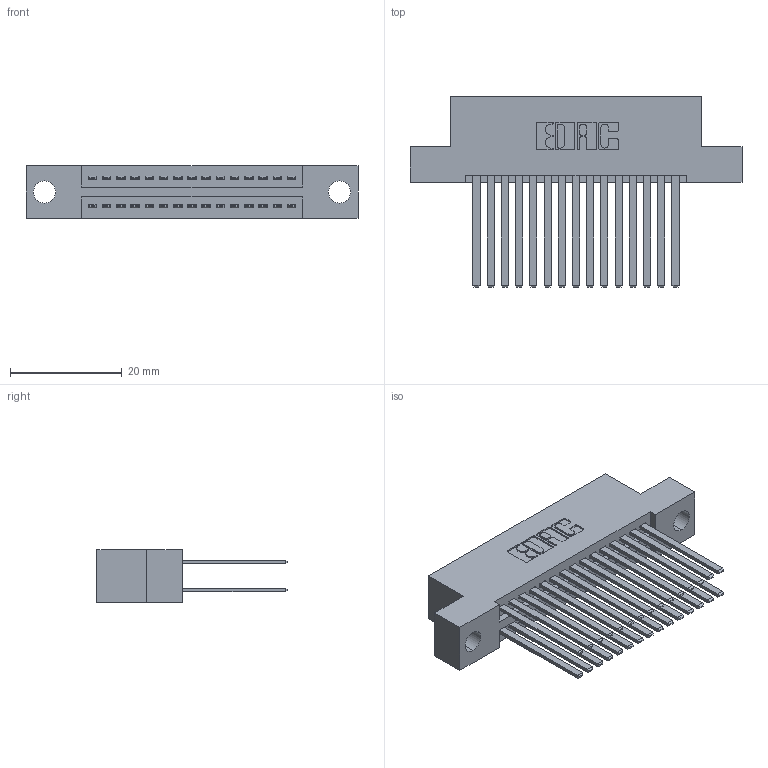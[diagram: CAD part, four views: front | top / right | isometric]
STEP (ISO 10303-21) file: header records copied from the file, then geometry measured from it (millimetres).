
FILE_DESCRIPTION (( 'STEP AP203' ), '1' );
FILE_NAME ('345-030-544-204.STEP', '2021-05-19T23:26:28', ( '' ), ( '' ), 'SwSTEP 2.0', 'SolidWorks 2020', '' );
FILE_SCHEMA (( 'CONFIG_CONTROL_DESIGN' ));
Length unit declared in the file: inch
Products named in the file (3): 345-292-001_345-293-144; 345 Part_Flush Mounting Lugs - 0.156 Dia-TI; 345-030-544-204
Assembly tree (31 placements, depth 2):
  345-030-544-204
    345 Part_Flush Mounting Lugs - 0.156 Dia-TI
    345-292-001_345-293-144  x30
Bounding box: 59.31 x 33.96 x 9.4 mm (x, y, z)
Volume: 5825.3 mm3; surface area: 9172 mm2
Topology: 31 solids, 31 shells, 1460 faces, 4307 edges, 2830 vertices
Faces by surface type: plane 964, cylinder 496
Entity records: 15639 total; most frequent: CARTESIAN_POINT 2650, ORIENTED_EDGE 2582, DIRECTION 2367, EDGE_CURVE 1291, LINE 1103, VECTOR 1103, VERTEX_POINT 858, AXIS2_PLACEMENT_3D 632
